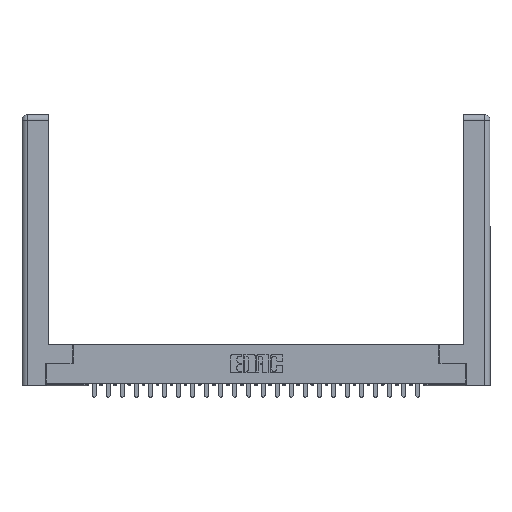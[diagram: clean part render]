
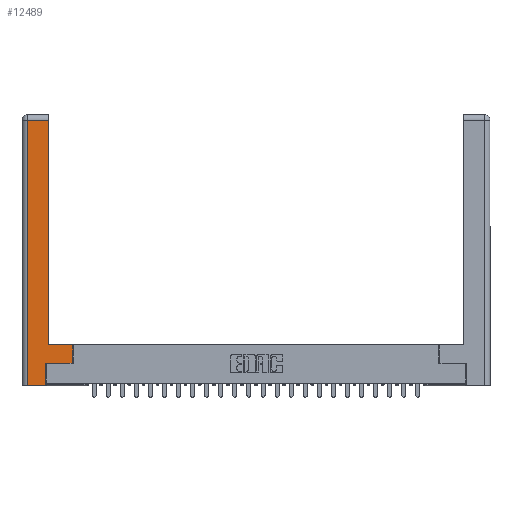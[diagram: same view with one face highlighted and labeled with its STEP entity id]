
A CAD part, top view. The second image highlights one B-rep face of the part: STEP entity #12489.
In plain terms, the highlighted planar face has unit normal (0, 0, 1).
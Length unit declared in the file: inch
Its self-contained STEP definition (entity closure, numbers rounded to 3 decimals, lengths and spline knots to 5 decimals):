
#383 = DIRECTION ( 'NONE',  ( 0., -1., 0. ) ) ;
#819 = ORIENTED_EDGE ( 'NONE', *, *, #14404, .T. ) ;
#1379 = ORIENTED_EDGE ( 'NONE', *, *, #8030, .T. ) ;
#1496 = ORIENTED_EDGE ( 'NONE', *, *, #28565, .T. ) ;
#2405 = LINE ( 'NONE', #21492, #8302 ) ;
#3131 = EDGE_CURVE ( 'NONE', #17689, #23601, #21247, .T. ) ;
#3433 = VERTEX_POINT ( 'NONE', #7853 ) ;
#3732 = LINE ( 'NONE', #9791, #29020 ) ;
#3911 = DIRECTION ( 'NONE',  ( 0., 1., 0. ) ) ;
#4661 = CARTESIAN_POINT ( 'NONE',  ( 0.265, 0.245, 0. ) ) ;
#4750 = VECTOR ( 'NONE', #8295, 39.37008 ) ;
#5195 = DIRECTION ( 'NONE',  ( 0., 0., -1. ) ) ;
#5796 = CARTESIAN_POINT ( 'NONE',  ( 0.0615, 2.94, 0. ) ) ;
#5908 = DIRECTION ( 'NONE',  ( -1., 0., 0. ) ) ;
#6583 = ORIENTED_EDGE ( 'NONE', *, *, #21965, .T. ) ;
#6637 = FACE_OUTER_BOUND ( 'NONE', #28846, .T. ) ;
#6665 = VECTOR ( 'NONE', #27922, 39.37008 ) ;
#7335 = VERTEX_POINT ( 'NONE', #17717 ) ;
#7347 = CARTESIAN_POINT ( 'NONE',  ( 0.265, 0., 0. ) ) ;
#7853 = CARTESIAN_POINT ( 'NONE',  ( 0.565, 0.245, 0. ) ) ;
#8030 = EDGE_CURVE ( 'NONE', #7335, #16072, #28086, .T. ) ;
#8232 = VERTEX_POINT ( 'NONE', #22187 ) ;
#8295 = DIRECTION ( 'NONE',  ( 0., 1., 0. ) ) ;
#8302 = VECTOR ( 'NONE', #383, 39.37008 ) ;
#8813 = EDGE_CURVE ( 'NONE', #23601, #3433, #16423, .T. ) ;
#9236 = EDGE_CURVE ( 'NONE', #16072, #30421, #2405, .T. ) ;
#9791 = CARTESIAN_POINT ( 'NONE',  ( 0.565, 0.45, 0. ) ) ;
#9913 = LINE ( 'NONE', #27261, #4750 ) ;
#9948 = LINE ( 'NONE', #13810, #6665 ) ;
#10162 = AXIS2_PLACEMENT_3D ( 'NONE', #17302, #5195, #14478 ) ;
#10903 = CARTESIAN_POINT ( 'NONE',  ( 0.565, 0.245, 0. ) ) ;
#12489 = ADVANCED_FACE ( 'NONE', ( #6637 ), #24126, .F. ) ;
#12768 = VECTOR ( 'NONE', #5908, 39.37008 ) ;
#13374 = ORIENTED_EDGE ( 'NONE', *, *, #8813, .T. ) ;
#13453 = VECTOR ( 'NONE', #17882, 39.37008 ) ;
#13810 = CARTESIAN_POINT ( 'NONE',  ( 0.295, 0.45, 0. ) ) ;
#14404 = EDGE_CURVE ( 'NONE', #3433, #8232, #3732, .T. ) ;
#14433 = CARTESIAN_POINT ( 'NONE',  ( 0.0615, 2.94, 0. ) ) ;
#14478 = DIRECTION ( 'NONE',  ( -1., 0., 0. ) ) ;
#15493 = CARTESIAN_POINT ( 'NONE',  ( 0.295, 0.45, 0. ) ) ;
#16072 = VERTEX_POINT ( 'NONE', #14433 ) ;
#16423 = LINE ( 'NONE', #10903, #13453 ) ;
#16660 = DIRECTION ( 'NONE',  ( 1., 0., 0. ) ) ;
#17302 = CARTESIAN_POINT ( 'NONE',  ( 0., 0., 0. ) ) ;
#17689 = VERTEX_POINT ( 'NONE', #29480 ) ;
#17717 = CARTESIAN_POINT ( 'NONE',  ( 0.295, 2.94, 0. ) ) ;
#17882 = DIRECTION ( 'NONE',  ( 1., 0., 0. ) ) ;
#18966 = ORIENTED_EDGE ( 'NONE', *, *, #27546, .T. ) ;
#19304 = VECTOR ( 'NONE', #16660, 39.37008 ) ;
#20493 = VERTEX_POINT ( 'NONE', #15493 ) ;
#21224 = LINE ( 'NONE', #7347, #19304 ) ;
#21247 = LINE ( 'NONE', #23196, #27217 ) ;
#21492 = CARTESIAN_POINT ( 'NONE',  ( 0.0615, 0., 0. ) ) ;
#21965 = EDGE_CURVE ( 'NONE', #20493, #7335, #9913, .T. ) ;
#22187 = CARTESIAN_POINT ( 'NONE',  ( 0.565, 0.45, 0. ) ) ;
#23196 = CARTESIAN_POINT ( 'NONE',  ( 0.265, 0.245, 0. ) ) ;
#23601 = VERTEX_POINT ( 'NONE', #4661 ) ;
#23653 = CARTESIAN_POINT ( 'NONE',  ( 0.0615, 0., 0. ) ) ;
#24126 = PLANE ( 'NONE',  #10162 ) ;
#25956 = ORIENTED_EDGE ( 'NONE', *, *, #9236, .T. ) ;
#27217 = VECTOR ( 'NONE', #3911, 39.37008 ) ;
#27261 = CARTESIAN_POINT ( 'NONE',  ( 0.295, 3., 0. ) ) ;
#27546 = EDGE_CURVE ( 'NONE', #30421, #17689, #21224, .T. ) ;
#27922 = DIRECTION ( 'NONE',  ( -1., 0., 0. ) ) ;
#28086 = LINE ( 'NONE', #5796, #12768 ) ;
#28565 = EDGE_CURVE ( 'NONE', #8232, #20493, #9948, .T. ) ;
#28770 = DIRECTION ( 'NONE',  ( 0., 1., 0. ) ) ;
#28846 = EDGE_LOOP ( 'NONE', ( #6583, #1379, #25956, #18966, #29188, #13374, #819, #1496 ) ) ;
#29020 = VECTOR ( 'NONE', #28770, 39.37008 ) ;
#29188 = ORIENTED_EDGE ( 'NONE', *, *, #3131, .T. ) ;
#29480 = CARTESIAN_POINT ( 'NONE',  ( 0.265, 0., 0. ) ) ;
#30421 = VERTEX_POINT ( 'NONE', #23653 ) ;
